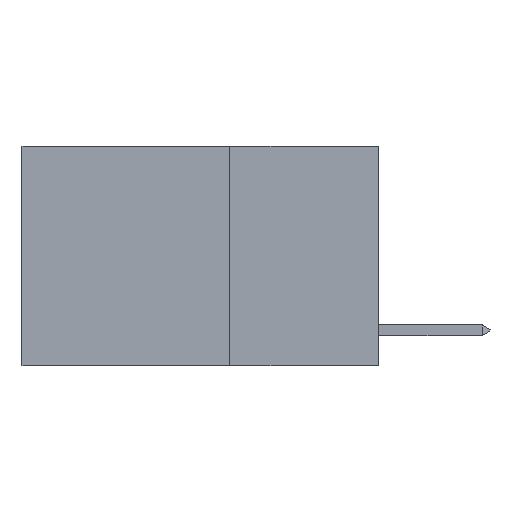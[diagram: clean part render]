
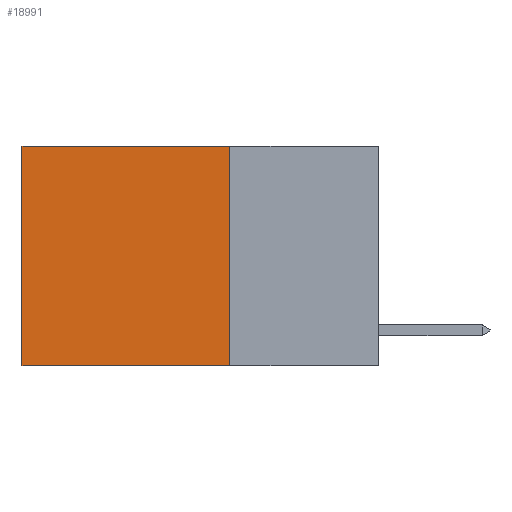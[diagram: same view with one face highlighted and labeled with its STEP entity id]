
A CAD part, left-side view. The second image highlights one B-rep face of the part: STEP entity #18991.
In plain terms, the highlighted planar face has unit normal (-1, 0, 0).
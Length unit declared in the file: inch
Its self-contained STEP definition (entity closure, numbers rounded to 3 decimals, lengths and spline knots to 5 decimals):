
#434 = LINE ( 'NONE', #9164, #11164 ) ;
#640 = DIRECTION ( 'NONE',  ( 0., 1., 0. ) ) ;
#1537 = VECTOR ( 'NONE', #22627, 39.37008 ) ;
#2048 = EDGE_CURVE ( 'NONE', #4881, #4821, #18012, .T. ) ;
#2266 = DIRECTION ( 'NONE',  ( 0., 0., -1. ) ) ;
#3416 = ORIENTED_EDGE ( 'NONE', *, *, #11024, .F. ) ;
#4475 = ORIENTED_EDGE ( 'NONE', *, *, #10823, .F. ) ;
#4479 = VECTOR ( 'NONE', #10215, 39.37008 ) ;
#4570 = CARTESIAN_POINT ( 'NONE',  ( 0.2625, 0.25, 0. ) ) ;
#4821 = VERTEX_POINT ( 'NONE', #15504 ) ;
#4881 = VERTEX_POINT ( 'NONE', #11256 ) ;
#5118 = VECTOR ( 'NONE', #640, 39.37008 ) ;
#5722 = ORIENTED_EDGE ( 'NONE', *, *, #14749, .T. ) ;
#6990 = LINE ( 'NONE', #8701, #1537 ) ;
#7640 = VERTEX_POINT ( 'NONE', #13128 ) ;
#7975 = CARTESIAN_POINT ( 'NONE',  ( 0.2625, 0.6, -0.37 ) ) ;
#8425 = DIRECTION ( 'NONE',  ( 1., 0., 0. ) ) ;
#8535 = PLANE ( 'NONE',  #17493 ) ;
#8562 = EDGE_LOOP ( 'NONE', ( #5722, #3416, #4475, #21302 ) ) ;
#8701 = CARTESIAN_POINT ( 'NONE',  ( 0.2625, 0.25, -0.37 ) ) ;
#9164 = CARTESIAN_POINT ( 'NONE',  ( 0.2625, 0.6, 0. ) ) ;
#10215 = DIRECTION ( 'NONE',  ( 0., 0., -1. ) ) ;
#10823 = EDGE_CURVE ( 'NONE', #4881, #7640, #18836, .T. ) ;
#11024 = EDGE_CURVE ( 'NONE', #7640, #18342, #6990, .T. ) ;
#11164 = VECTOR ( 'NONE', #2266, 39.37008 ) ;
#11256 = CARTESIAN_POINT ( 'NONE',  ( 0.2625, 0.25, 0. ) ) ;
#11863 = FACE_OUTER_BOUND ( 'NONE', #8562, .T. ) ;
#13128 = CARTESIAN_POINT ( 'NONE',  ( 0.2625, 0.25, -0.37 ) ) ;
#14749 = EDGE_CURVE ( 'NONE', #4821, #18342, #434, .T. ) ;
#15433 = DIRECTION ( 'NONE',  ( 0., 0., -1. ) ) ;
#15504 = CARTESIAN_POINT ( 'NONE',  ( 0.2625, 0.6, 0. ) ) ;
#16390 = CARTESIAN_POINT ( 'NONE',  ( 0.2625, 0.25, 0. ) ) ;
#17493 = AXIS2_PLACEMENT_3D ( 'NONE', #18884, #8425, #15433 ) ;
#18012 = LINE ( 'NONE', #16390, #5118 ) ;
#18342 = VERTEX_POINT ( 'NONE', #7975 ) ;
#18836 = LINE ( 'NONE', #4570, #4479 ) ;
#18884 = CARTESIAN_POINT ( 'NONE',  ( 0.2625, 0.25, 0. ) ) ;
#18991 = ADVANCED_FACE ( 'NONE', ( #11863 ), #8535, .F. ) ;
#21302 = ORIENTED_EDGE ( 'NONE', *, *, #2048, .T. ) ;
#22627 = DIRECTION ( 'NONE',  ( 0., 1., 0. ) ) ;
